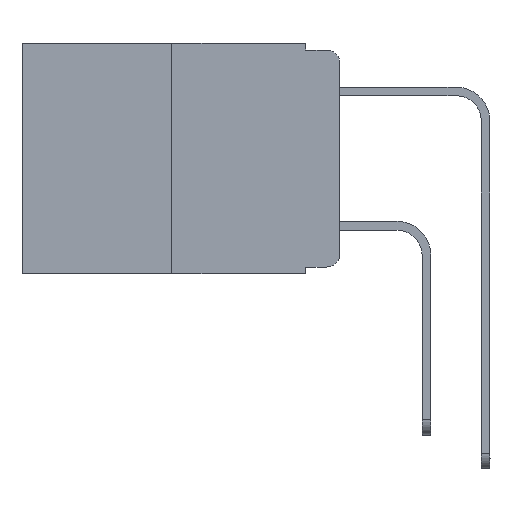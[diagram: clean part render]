
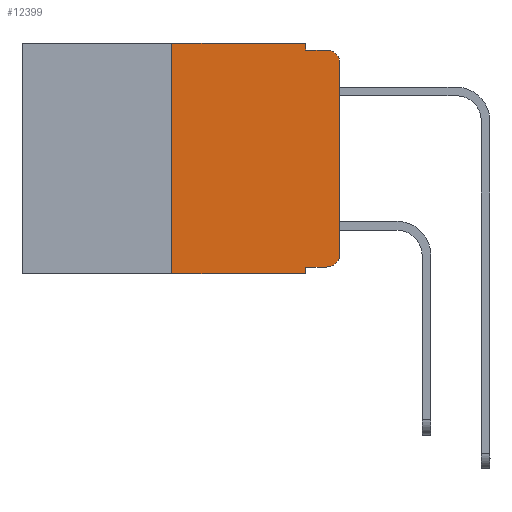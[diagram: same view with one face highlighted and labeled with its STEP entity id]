
A CAD part, left-side view. The second image highlights one B-rep face of the part: STEP entity #12399.
In plain terms, the highlighted planar face has unit normal (-1, 0, 0).
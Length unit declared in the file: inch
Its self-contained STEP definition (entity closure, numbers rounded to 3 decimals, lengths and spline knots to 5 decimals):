
#51 = CARTESIAN_POINT ( 'NONE',  ( 0., 0.25, 0. ) ) ;
#882 = DIRECTION ( 'NONE',  ( 0., 0., -1. ) ) ;
#1107 = DIRECTION ( 'NONE',  ( -1., 0., 0. ) ) ;
#1225 = PLANE ( 'NONE',  #18395 ) ;
#1590 = ORIENTED_EDGE ( 'NONE', *, *, #16146, .T. ) ;
#1829 = CARTESIAN_POINT ( 'NONE',  ( 0., 0.473, 0. ) ) ;
#1931 = CARTESIAN_POINT ( 'NONE',  ( 0., 0.051, -0.01 ) ) ;
#2153 = CARTESIAN_POINT ( 'NONE',  ( 0., 0., 0. ) ) ;
#2800 = VERTEX_POINT ( 'NONE', #17443 ) ;
#3707 = EDGE_CURVE ( 'NONE', #7475, #12856, #19264, .T. ) ;
#3757 = CARTESIAN_POINT ( 'NONE',  ( 0., 0.051, 0. ) ) ;
#3793 = LINE ( 'NONE', #2153, #5329 ) ;
#3936 = DIRECTION ( 'NONE',  ( 0., 0., -1. ) ) ;
#4161 = AXIS2_PLACEMENT_3D ( 'NONE', #14877, #18554, #5121 ) ;
#4886 = ORIENTED_EDGE ( 'NONE', *, *, #16843, .T. ) ;
#5121 = DIRECTION ( 'NONE',  ( 0., 0., -1. ) ) ;
#5329 = VECTOR ( 'NONE', #19108, 39.37008 ) ;
#5377 = LINE ( 'NONE', #16905, #11738 ) ;
#5412 = CARTESIAN_POINT ( 'NONE',  ( 0., 0.02, -0.333 ) ) ;
#6292 = DIRECTION ( 'NONE',  ( 0., 0., -1. ) ) ;
#6323 = VECTOR ( 'NONE', #15823, 39.37008 ) ;
#6560 = CARTESIAN_POINT ( 'NONE',  ( 0., 0.25, 0. ) ) ;
#6565 = ORIENTED_EDGE ( 'NONE', *, *, #7890, .F. ) ;
#6930 = EDGE_CURVE ( 'NONE', #12856, #21486, #19854, .T. ) ;
#7130 = DIRECTION ( 'NONE',  ( 0., -1., 0. ) ) ;
#7222 = VERTEX_POINT ( 'NONE', #8630 ) ;
#7475 = VERTEX_POINT ( 'NONE', #20043 ) ;
#7635 = EDGE_CURVE ( 'NONE', #7475, #14277, #12361, .T. ) ;
#7744 = EDGE_LOOP ( 'NONE', ( #19631, #4886, #19221, #6565, #15988, #11242, #1590, #11620, #19058, #10196 ) ) ;
#7890 = EDGE_CURVE ( 'NONE', #13830, #7222, #5377, .T. ) ;
#7944 = EDGE_CURVE ( 'NONE', #2800, #20790, #15244, .T. ) ;
#7967 = CARTESIAN_POINT ( 'NONE',  ( 0., 0.473, 0. ) ) ;
#8123 = VECTOR ( 'NONE', #10012, 39.37008 ) ;
#8579 = DIRECTION ( 'NONE',  ( 0., 0., -1. ) ) ;
#8630 = CARTESIAN_POINT ( 'NONE',  ( 0., 0.051, -0.01 ) ) ;
#9913 = AXIS2_PLACEMENT_3D ( 'NONE', #12632, #1107, #882 ) ;
#10012 = DIRECTION ( 'NONE',  ( 0., -1., 0. ) ) ;
#10196 = ORIENTED_EDGE ( 'NONE', *, *, #6930, .T. ) ;
#10875 = CARTESIAN_POINT ( 'NONE',  ( 0., 0.02, -0.01 ) ) ;
#11242 = ORIENTED_EDGE ( 'NONE', *, *, #7944, .F. ) ;
#11586 = CIRCLE ( 'NONE', #4161, 0.02 ) ;
#11620 = ORIENTED_EDGE ( 'NONE', *, *, #7635, .F. ) ;
#11738 = VECTOR ( 'NONE', #8579, 39.37008 ) ;
#11936 = CARTESIAN_POINT ( 'NONE',  ( 0., 0., -0.313 ) ) ;
#12246 = LINE ( 'NONE', #20916, #21685 ) ;
#12361 = LINE ( 'NONE', #21051, #15272 ) ;
#12399 = ADVANCED_FACE ( 'NONE', ( #14857 ), #1225, .F. ) ;
#12632 = CARTESIAN_POINT ( 'NONE',  ( 0., 0.02, -0.313 ) ) ;
#12856 = VERTEX_POINT ( 'NONE', #5412 ) ;
#13458 = EDGE_CURVE ( 'NONE', #21486, #15295, #3793, .T. ) ;
#13830 = VERTEX_POINT ( 'NONE', #3757 ) ;
#14277 = VERTEX_POINT ( 'NONE', #20303 ) ;
#14857 = FACE_OUTER_BOUND ( 'NONE', #7744, .T. ) ;
#14877 = CARTESIAN_POINT ( 'NONE',  ( 0., 0.02, -0.03 ) ) ;
#15244 = LINE ( 'NONE', #51, #17778 ) ;
#15272 = VECTOR ( 'NONE', #3936, 39.37008 ) ;
#15295 = VERTEX_POINT ( 'NONE', #20688 ) ;
#15571 = DIRECTION ( 'NONE',  ( 0., 0., 1. ) ) ;
#15823 = DIRECTION ( 'NONE',  ( 0., -1., 0. ) ) ;
#15988 = ORIENTED_EDGE ( 'NONE', *, *, #17694, .F. ) ;
#16146 = EDGE_CURVE ( 'NONE', #2800, #14277, #12246, .T. ) ;
#16239 = VECTOR ( 'NONE', #20369, 39.37008 ) ;
#16843 = EDGE_CURVE ( 'NONE', #15295, #20447, #11586, .T. ) ;
#16905 = CARTESIAN_POINT ( 'NONE',  ( 0., 0.051, 0. ) ) ;
#17443 = CARTESIAN_POINT ( 'NONE',  ( 0., 0.25, -0.343 ) ) ;
#17494 = CARTESIAN_POINT ( 'NONE',  ( 0., 0.051, -0.333 ) ) ;
#17694 = EDGE_CURVE ( 'NONE', #20790, #13830, #18580, .T. ) ;
#17778 = VECTOR ( 'NONE', #15571, 39.37008 ) ;
#18395 = AXIS2_PLACEMENT_3D ( 'NONE', #7967, #21543, #6292 ) ;
#18554 = DIRECTION ( 'NONE',  ( -1., 0., 0. ) ) ;
#18580 = LINE ( 'NONE', #1829, #16239 ) ;
#19058 = ORIENTED_EDGE ( 'NONE', *, *, #3707, .T. ) ;
#19108 = DIRECTION ( 'NONE',  ( 0., 0., 1. ) ) ;
#19221 = ORIENTED_EDGE ( 'NONE', *, *, #20785, .F. ) ;
#19264 = LINE ( 'NONE', #17494, #6323 ) ;
#19631 = ORIENTED_EDGE ( 'NONE', *, *, #13458, .T. ) ;
#19854 = CIRCLE ( 'NONE', #9913, 0.02 ) ;
#20043 = CARTESIAN_POINT ( 'NONE',  ( 0., 0.051, -0.333 ) ) ;
#20303 = CARTESIAN_POINT ( 'NONE',  ( 0., 0.051, -0.343 ) ) ;
#20369 = DIRECTION ( 'NONE',  ( 0., -1., 0. ) ) ;
#20447 = VERTEX_POINT ( 'NONE', #10875 ) ;
#20470 = LINE ( 'NONE', #1931, #8123 ) ;
#20688 = CARTESIAN_POINT ( 'NONE',  ( 0., 0., -0.03 ) ) ;
#20785 = EDGE_CURVE ( 'NONE', #7222, #20447, #20470, .T. ) ;
#20790 = VERTEX_POINT ( 'NONE', #6560 ) ;
#20916 = CARTESIAN_POINT ( 'NONE',  ( 0., 0.473, -0.343 ) ) ;
#21051 = CARTESIAN_POINT ( 'NONE',  ( 0., 0.051, 0. ) ) ;
#21486 = VERTEX_POINT ( 'NONE', #11936 ) ;
#21543 = DIRECTION ( 'NONE',  ( 1., 0., 0. ) ) ;
#21685 = VECTOR ( 'NONE', #7130, 39.37008 ) ;
